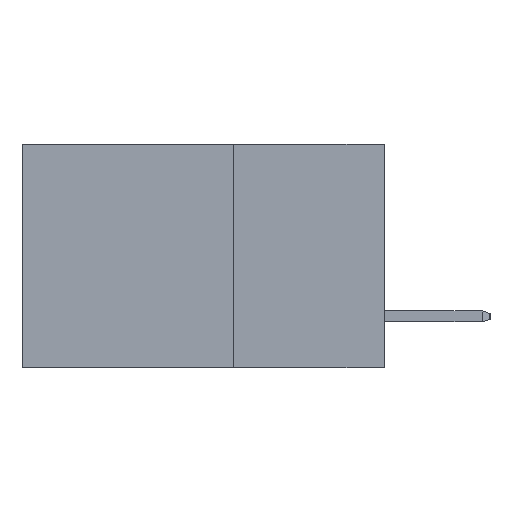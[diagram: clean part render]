
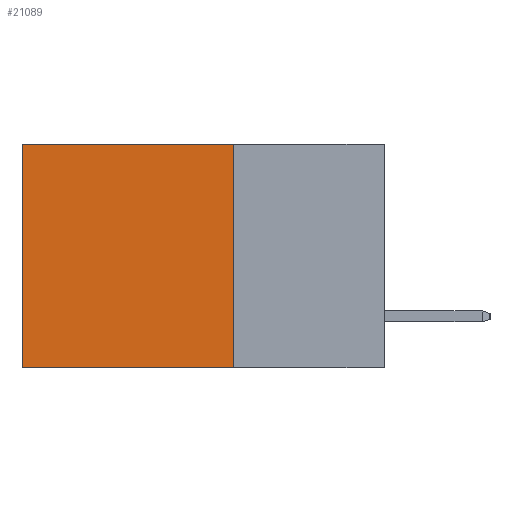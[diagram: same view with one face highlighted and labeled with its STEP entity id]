
A CAD part, left-side view. The second image highlights one B-rep face of the part: STEP entity #21089.
In plain terms, the highlighted planar face has unit normal (-1, 0, 0).
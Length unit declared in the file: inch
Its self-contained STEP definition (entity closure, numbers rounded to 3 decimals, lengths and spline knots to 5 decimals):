
#492 = VECTOR ( 'NONE', #16393, 39.37008 ) ;
#1649 = EDGE_CURVE ( 'NONE', #16338, #7240, #17489, .T. ) ;
#2053 = DIRECTION ( 'NONE',  ( 0., 0., -1. ) ) ;
#2082 = CARTESIAN_POINT ( 'NONE',  ( 0.298, 0.6, 0. ) ) ;
#2626 = EDGE_CURVE ( 'NONE', #7240, #4972, #5603, .T. ) ;
#2889 = ORIENTED_EDGE ( 'NONE', *, *, #3187, .T. ) ;
#3187 = EDGE_CURVE ( 'NONE', #14431, #4972, #22172, .T. ) ;
#3993 = CARTESIAN_POINT ( 'NONE',  ( 0.298, 0.25, -0.37 ) ) ;
#4972 = VERTEX_POINT ( 'NONE', #12431 ) ;
#5603 = LINE ( 'NONE', #22556, #492 ) ;
#5693 = CARTESIAN_POINT ( 'NONE',  ( 0.298, 0.25, 0. ) ) ;
#6262 = PLANE ( 'NONE',  #19470 ) ;
#7240 = VERTEX_POINT ( 'NONE', #3993 ) ;
#8800 = VECTOR ( 'NONE', #20842, 39.37008 ) ;
#8886 = DIRECTION ( 'NONE',  ( 0., 0., -1. ) ) ;
#9253 = ORIENTED_EDGE ( 'NONE', *, *, #15140, .T. ) ;
#9407 = LINE ( 'NONE', #5693, #8800 ) ;
#10066 = DIRECTION ( 'NONE',  ( 1., 0., 0. ) ) ;
#12431 = CARTESIAN_POINT ( 'NONE',  ( 0.298, 0.6, -0.37 ) ) ;
#12439 = VECTOR ( 'NONE', #8886, 39.37008 ) ;
#13788 = CARTESIAN_POINT ( 'NONE',  ( 0.298, 0.25, 0. ) ) ;
#13827 = VECTOR ( 'NONE', #2053, 39.37008 ) ;
#14431 = VERTEX_POINT ( 'NONE', #14904 ) ;
#14810 = CARTESIAN_POINT ( 'NONE',  ( 0.298, 0.25, 0. ) ) ;
#14904 = CARTESIAN_POINT ( 'NONE',  ( 0.298, 0.6, 0. ) ) ;
#15140 = EDGE_CURVE ( 'NONE', #16338, #14431, #9407, .T. ) ;
#16338 = VERTEX_POINT ( 'NONE', #21209 ) ;
#16393 = DIRECTION ( 'NONE',  ( 0., 1., 0. ) ) ;
#17489 = LINE ( 'NONE', #14810, #12439 ) ;
#18799 = EDGE_LOOP ( 'NONE', ( #2889, #23900, #24136, #9253 ) ) ;
#19470 = AXIS2_PLACEMENT_3D ( 'NONE', #13788, #10066, #23308 ) ;
#20842 = DIRECTION ( 'NONE',  ( 0., 1., 0. ) ) ;
#21089 = ADVANCED_FACE ( 'NONE', ( #23990 ), #6262, .F. ) ;
#21209 = CARTESIAN_POINT ( 'NONE',  ( 0.298, 0.25, 0. ) ) ;
#22172 = LINE ( 'NONE', #2082, #13827 ) ;
#22556 = CARTESIAN_POINT ( 'NONE',  ( 0.298, 0.25, -0.37 ) ) ;
#23308 = DIRECTION ( 'NONE',  ( 0., 0., -1. ) ) ;
#23900 = ORIENTED_EDGE ( 'NONE', *, *, #2626, .F. ) ;
#23990 = FACE_OUTER_BOUND ( 'NONE', #18799, .T. ) ;
#24136 = ORIENTED_EDGE ( 'NONE', *, *, #1649, .F. ) ;
